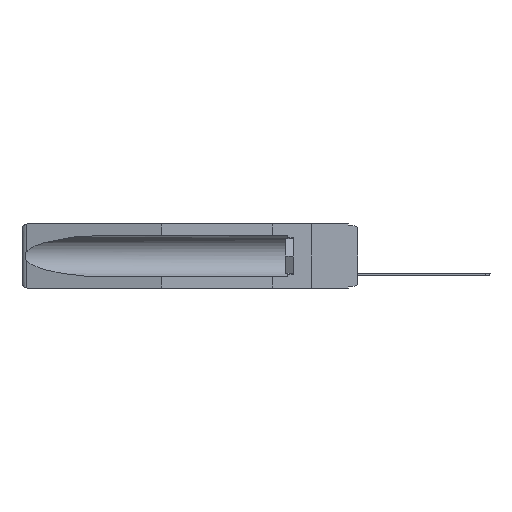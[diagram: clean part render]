
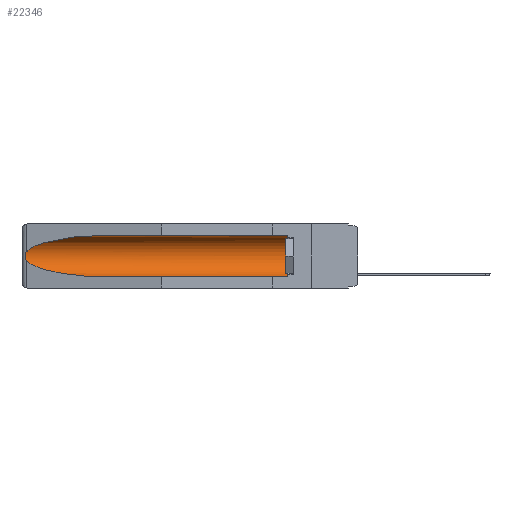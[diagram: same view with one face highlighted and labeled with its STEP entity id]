
A CAD part, left-side view. The second image highlights one B-rep face of the part: STEP entity #22346.
In plain terms, the highlighted cylindrical face has radius 2.857 mm (diameter 5.715 mm), a partial arc.
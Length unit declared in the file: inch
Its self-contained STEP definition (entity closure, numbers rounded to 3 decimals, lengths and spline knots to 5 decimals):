
#190 = ORIENTED_EDGE ( 'NONE', *, *, #8874, .T. ) ;
#265 = EDGE_CURVE ( 'NONE', #2483, #9952, #4698, .T. ) ;
#998 = CARTESIAN_POINT ( 'NONE',  ( 0.26597, 1.5296, -0.19026 ) ) ;
#1033 = AXIS2_PLACEMENT_3D ( 'NONE', #25502, #8978, #21441 ) ;
#1118 = CARTESIAN_POINT ( 'NONE',  ( 0.2675, 1.53308, -0.17534 ) ) ;
#1245 = CARTESIAN_POINT ( 'NONE',  ( 0.26537, 1.52718, -0.14972 ) ) ;
#2057 = EDGE_CURVE ( 'NONE', #9952, #17054, #9379, .T. ) ;
#2483 = VERTEX_POINT ( 'NONE', #4868 ) ;
#4559 = ORIENTED_EDGE ( 'NONE', *, *, #265, .T. ) ;
#4698 = LINE ( 'NONE', #16518, #19397 ) ;
#4868 = CARTESIAN_POINT ( 'NONE',  ( 0.155, 0.126, -0.059 ) ) ;
#5494 = CIRCLE ( 'NONE', #20156, 0.1125 ) ;
#6886 = CARTESIAN_POINT ( 'NONE',  ( 0.155, 1.07973, -0.059 ) ) ;
#6903 = CARTESIAN_POINT ( 'NONE',  ( 0.2673, 1.53269, -0.17917 ) ) ;
#7035 = B_SPLINE_CURVE_WITH_KNOTS ( 'NONE', 3,
 ( #1245, #9255, #24747, #20806, #21323, #1118, #6903, #16888, #998, #25002 ),
 .UNSPECIFIED., .F., .F.,
 ( 4, 2, 2, 2, 4 ),
 ( 0., 0.00029, 0.00058, 0.00087, 0.00117 ),
 .UNSPECIFIED. ) ;
#8229 = CARTESIAN_POINT ( 'NONE',  ( 0.155, 0.126, -0.1715 ) ) ;
#8874 = EDGE_CURVE ( 'NONE', #19544, #17921, #20107, .T. ) ;
#8978 = DIRECTION ( 'NONE',  ( 0., 1., 0. ) ) ;
#9255 = CARTESIAN_POINT ( 'NONE',  ( 0.26597, 1.52961, -0.15275 ) ) ;
#9379 =( BOUNDED_CURVE ( )  B_SPLINE_CURVE ( 3, ( #6886, #14877, #20921, #22878 ),
 .UNSPECIFIED., .F., .T. ) 
 B_SPLINE_CURVE_WITH_KNOTS ( ( 4, 4 ),
 ( 4.71239, 6.08839 ),
 .UNSPECIFIED. ) 
 CURVE ( )  GEOMETRIC_REPRESENTATION_ITEM ( )  RATIONAL_B_SPLINE_CURVE ( ( 1., 0.848, 0.848, 1. ) ) 
 REPRESENTATION_ITEM ( '' )  );
#9649 = ORIENTED_EDGE ( 'NONE', *, *, #12892, .T. ) ;
#9952 = VERTEX_POINT ( 'NONE', #24791 ) ;
#10315 = DIRECTION ( 'NONE',  ( 0., 0., 1. ) ) ;
#10600 = DIRECTION ( 'NONE',  ( 0., 1., 0. ) ) ;
#11098 = CARTESIAN_POINT ( 'NONE',  ( 0.25451, 1.48313, -0.24835 ) ) ;
#12414 = CARTESIAN_POINT ( 'NONE',  ( 0.155, 0.126, -0.284 ) ) ;
#12892 = EDGE_CURVE ( 'NONE', #21860, #2483, #5494, .T. ) ;
#13135 = CARTESIAN_POINT ( 'NONE',  ( 0.155, 1.07973, -0.284 ) ) ;
#14374 = VECTOR ( 'NONE', #19668, 39.37008 ) ;
#14519 = ORIENTED_EDGE ( 'NONE', *, *, #19828, .F. ) ;
#14733 = CARTESIAN_POINT ( 'NONE',  ( 0.155, 1.07973, -0.284 ) ) ;
#14877 = CARTESIAN_POINT ( 'NONE',  ( 0.21114, 1.30732, -0.059 ) ) ;
#16232 = DIRECTION ( 'NONE',  ( 0., -1., 0. ) ) ;
#16518 = CARTESIAN_POINT ( 'NONE',  ( 0.155, -0.30754, -0.059 ) ) ;
#16888 = CARTESIAN_POINT ( 'NONE',  ( 0.26655, 1.53094, -0.18657 ) ) ;
#17054 = VERTEX_POINT ( 'NONE', #20484 ) ;
#17502 = CYLINDRICAL_SURFACE ( 'NONE', #1033, 0.1125 ) ;
#17840 = LINE ( 'NONE', #21636, #14374 ) ;
#17921 = VERTEX_POINT ( 'NONE', #13135 ) ;
#19120 = CARTESIAN_POINT ( 'NONE',  ( 0.21114, 1.30732, -0.284 ) ) ;
#19397 = VECTOR ( 'NONE', #10600, 39.37008 ) ;
#19544 = VERTEX_POINT ( 'NONE', #22439 ) ;
#19668 = DIRECTION ( 'NONE',  ( 0., 1., 0. ) ) ;
#19828 = EDGE_CURVE ( 'NONE', #21860, #17921, #17840, .T. ) ;
#20107 =( BOUNDED_CURVE ( )  B_SPLINE_CURVE ( 3, ( #21083, #11098, #19120, #14733 ),
 .UNSPECIFIED., .F., .F. ) 
 B_SPLINE_CURVE_WITH_KNOTS ( ( 4, 4 ),
 ( 0.1948, 1.5708 ),
 .UNSPECIFIED. ) 
 CURVE ( )  GEOMETRIC_REPRESENTATION_ITEM ( )  RATIONAL_B_SPLINE_CURVE ( ( 1., 0.848, 0.848, 1. ) ) 
 REPRESENTATION_ITEM ( '' )  );
#20156 = AXIS2_PLACEMENT_3D ( 'NONE', #8229, #16232, #10315 ) ;
#20230 = ORIENTED_EDGE ( 'NONE', *, *, #2057, .T. ) ;
#20484 = CARTESIAN_POINT ( 'NONE',  ( 0.26537, 1.52718, -0.14972 ) ) ;
#20806 = CARTESIAN_POINT ( 'NONE',  ( 0.2673, 1.5327, -0.16383 ) ) ;
#20921 = CARTESIAN_POINT ( 'NONE',  ( 0.25451, 1.48313, -0.09465 ) ) ;
#21083 = CARTESIAN_POINT ( 'NONE',  ( 0.26537, 1.52718, -0.19328 ) ) ;
#21323 = CARTESIAN_POINT ( 'NONE',  ( 0.2675, 1.53308, -0.16763 ) ) ;
#21441 = DIRECTION ( 'NONE',  ( 0., 0., 1. ) ) ;
#21517 = ORIENTED_EDGE ( 'NONE', *, *, #25708, .T. ) ;
#21636 = CARTESIAN_POINT ( 'NONE',  ( 0.155, -0.30754, -0.284 ) ) ;
#21860 = VERTEX_POINT ( 'NONE', #12414 ) ;
#22346 = ADVANCED_FACE ( 'NONE', ( #23391 ), #17502, .F. ) ;
#22439 = CARTESIAN_POINT ( 'NONE',  ( 0.26537, 1.52718, -0.19328 ) ) ;
#22878 = CARTESIAN_POINT ( 'NONE',  ( 0.26537, 1.52718, -0.14972 ) ) ;
#23391 = FACE_OUTER_BOUND ( 'NONE', #25967, .T. ) ;
#24747 = CARTESIAN_POINT ( 'NONE',  ( 0.26654, 1.53092, -0.15636 ) ) ;
#24791 = CARTESIAN_POINT ( 'NONE',  ( 0.155, 1.07973, -0.059 ) ) ;
#25002 = CARTESIAN_POINT ( 'NONE',  ( 0.26537, 1.52718, -0.19328 ) ) ;
#25502 = CARTESIAN_POINT ( 'NONE',  ( 0.155, -0.30754, -0.1715 ) ) ;
#25708 = EDGE_CURVE ( 'NONE', #17054, #19544, #7035, .T. ) ;
#25967 = EDGE_LOOP ( 'NONE', ( #20230, #21517, #190, #14519, #9649, #4559 ) ) ;
